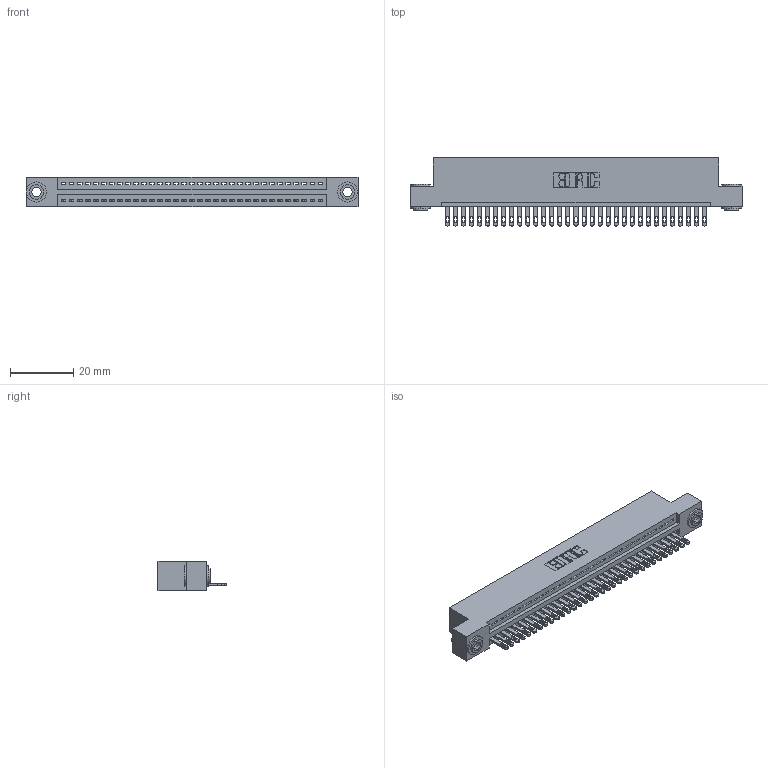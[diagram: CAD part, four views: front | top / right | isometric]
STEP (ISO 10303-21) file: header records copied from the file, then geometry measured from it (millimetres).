
FILE_DESCRIPTION (( 'STEP AP203' ), '1' );
FILE_NAME ('895-033-500-103.STEP', '2020-09-25T20:21:46', ( '' ), ( '' ), 'SwSTEP 2.0', 'SolidWorks 2020', '' );
FILE_SCHEMA (( 'CONFIG_CONTROL_DESIGN' ));
Length unit declared in the file: inch
Products named in the file (4): 845 Part_Flush Mounting Lugs - 0.156 Dia-TH; 345-250-002_345-250-002-102; 895-033-500-103; 345-292-001_345-293-100
Assembly tree (36 placements, depth 2):
  895-033-500-103
    845 Part_Flush Mounting Lugs - 0.156 Dia-TH
    345-292-001_345-293-100  x33
    345-250-002_345-250-002-102  x2
Bounding box: 105.03 x 21.51 x 9.4 mm (x, y, z)
Volume: 9941.9 mm3; surface area: 13378.1 mm2
Topology: 36 solids, 36 shells, 1946 faces, 5961 edges, 3970 vertices
Faces by surface type: plane 1212, cylinder 726, cone 8
Entity records: 26628 total; most frequent: CARTESIAN_POINT 4590, ORIENTED_EDGE 4550, DIRECTION 4055, EDGE_CURVE 2275, LINE 1983, VECTOR 1983, VERTEX_POINT 1514, AXIS2_PLACEMENT_3D 1036
